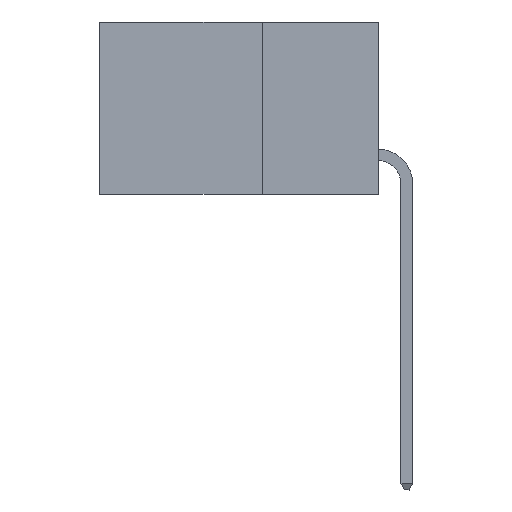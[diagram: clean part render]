
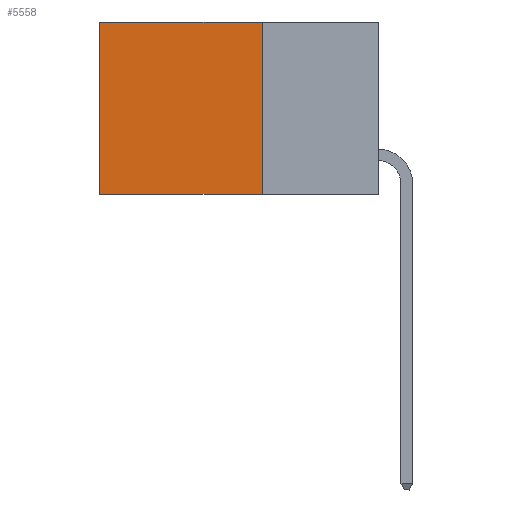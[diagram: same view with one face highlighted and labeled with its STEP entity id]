
A CAD part, left-side view. The second image highlights one B-rep face of the part: STEP entity #5558.
In plain terms, the highlighted planar face has unit normal (-1, 0, 0).
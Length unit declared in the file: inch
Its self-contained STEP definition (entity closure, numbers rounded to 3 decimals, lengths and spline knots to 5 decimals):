
#90 = LINE ( 'NONE', #3315, #392 ) ;
#392 = VECTOR ( 'NONE', #9024, 39.37008 ) ;
#894 = DIRECTION ( 'NONE',  ( 0., 0., -1. ) ) ;
#971 = ORIENTED_EDGE ( 'NONE', *, *, #10383, .F. ) ;
#1033 = CARTESIAN_POINT ( 'NONE',  ( 0.298, 0.25, 0. ) ) ;
#1090 = DIRECTION ( 'NONE',  ( 1., 0., 0. ) ) ;
#1236 = CARTESIAN_POINT ( 'NONE',  ( 0.298, 0.25, 0. ) ) ;
#1637 = LINE ( 'NONE', #11014, #8118 ) ;
#2081 = PLANE ( 'NONE',  #4288 ) ;
#2305 = ORIENTED_EDGE ( 'NONE', *, *, #9635, .F. ) ;
#2381 = VERTEX_POINT ( 'NONE', #8630 ) ;
#2699 = VERTEX_POINT ( 'NONE', #2995 ) ;
#2804 = FACE_OUTER_BOUND ( 'NONE', #10948, .T. ) ;
#2995 = CARTESIAN_POINT ( 'NONE',  ( 0.298, 0.25, -0.37 ) ) ;
#3315 = CARTESIAN_POINT ( 'NONE',  ( 0.298, 0.25, 0. ) ) ;
#4235 = VERTEX_POINT ( 'NONE', #4574 ) ;
#4288 = AXIS2_PLACEMENT_3D ( 'NONE', #1033, #1090, #8153 ) ;
#4574 = CARTESIAN_POINT ( 'NONE',  ( 0.298, 0.6, -0.37 ) ) ;
#5529 = VERTEX_POINT ( 'NONE', #1236 ) ;
#5558 = ADVANCED_FACE ( 'NONE', ( #2804 ), #2081, .F. ) ;
#5626 = LINE ( 'NONE', #10113, #7466 ) ;
#6388 = CARTESIAN_POINT ( 'NONE',  ( 0.298, 0.25, -0.37 ) ) ;
#6941 = ORIENTED_EDGE ( 'NONE', *, *, #10558, .T. ) ;
#7202 = DIRECTION ( 'NONE',  ( 0., 1., 0. ) ) ;
#7466 = VECTOR ( 'NONE', #10102, 39.37008 ) ;
#8089 = EDGE_CURVE ( 'NONE', #2381, #4235, #5626, .T. ) ;
#8118 = VECTOR ( 'NONE', #894, 39.37008 ) ;
#8153 = DIRECTION ( 'NONE',  ( 0., 0., -1. ) ) ;
#8212 = ORIENTED_EDGE ( 'NONE', *, *, #8089, .T. ) ;
#8630 = CARTESIAN_POINT ( 'NONE',  ( 0.298, 0.6, 0. ) ) ;
#8874 = LINE ( 'NONE', #6388, #10783 ) ;
#9024 = DIRECTION ( 'NONE',  ( 0., 1., 0. ) ) ;
#9635 = EDGE_CURVE ( 'NONE', #5529, #2699, #1637, .T. ) ;
#10102 = DIRECTION ( 'NONE',  ( 0., 0., -1. ) ) ;
#10113 = CARTESIAN_POINT ( 'NONE',  ( 0.298, 0.6, 0. ) ) ;
#10383 = EDGE_CURVE ( 'NONE', #2699, #4235, #8874, .T. ) ;
#10558 = EDGE_CURVE ( 'NONE', #5529, #2381, #90, .T. ) ;
#10783 = VECTOR ( 'NONE', #7202, 39.37008 ) ;
#10948 = EDGE_LOOP ( 'NONE', ( #8212, #971, #2305, #6941 ) ) ;
#11014 = CARTESIAN_POINT ( 'NONE',  ( 0.298, 0.25, 0. ) ) ;
